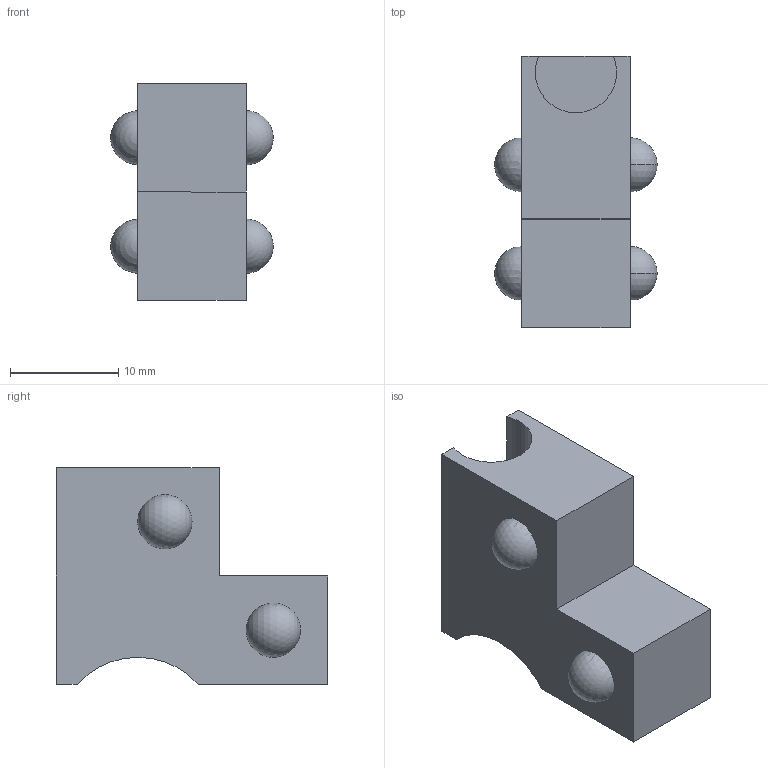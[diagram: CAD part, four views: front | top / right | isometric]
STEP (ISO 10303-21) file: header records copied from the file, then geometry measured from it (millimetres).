
FILE_DESCRIPTION (( 'STEP AP214' ), '1' );
FILE_NAME ('Bottom_Shaft_Holder.STEP', '2013-11-21T02:43:49', ( '' ), ( '' ), 'SwSTEP 2.0', 'SolidWorks 2013', '' );
FILE_SCHEMA (( 'AUTOMOTIVE_DESIGN' ));
Length unit declared in the file: millimetre
Products named in the file (1): Bottom_Shaft_Holder
Bounding box: 14.98 x 25 x 20 mm (x, y, z)
Volume: 3609.3 mm3; surface area: 1833.1 mm2
Topology: 1 solids, 1 shells, 21 faces, 65 edges, 42 vertices
Faces by surface type: plane 10, sphere 6, cylinder 5
Entity records: 649 total; most frequent: DIRECTION 113, CARTESIAN_POINT 105, ORIENTED_EDGE 98, EDGE_CURVE 49, AXIS2_PLACEMENT_3D 42, VERTEX_POINT 34, VECTOR 29, LINE 29
